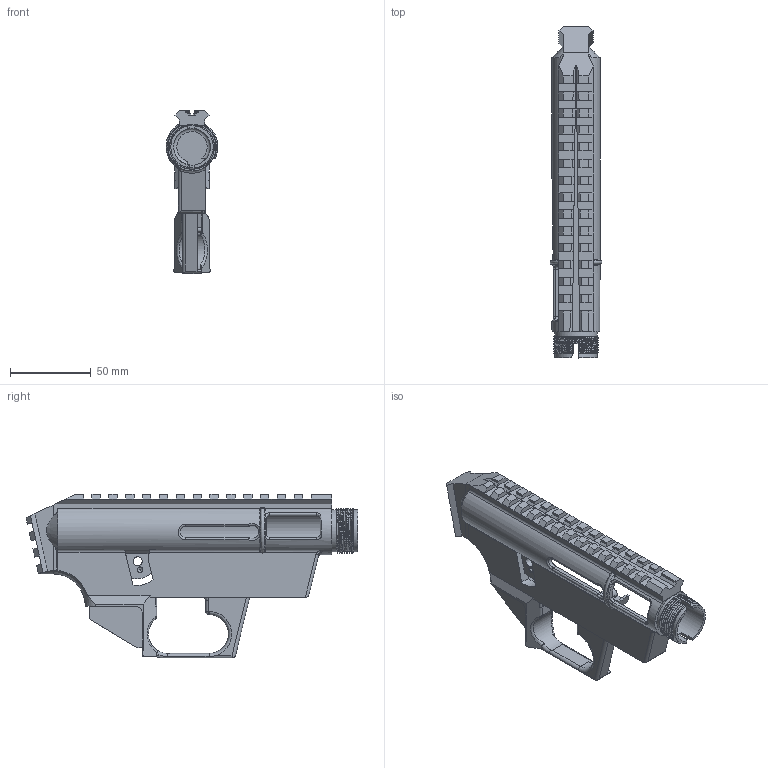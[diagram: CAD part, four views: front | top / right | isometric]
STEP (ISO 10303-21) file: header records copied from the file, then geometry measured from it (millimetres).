
FILE_DESCRIPTION(/* description */ (''),/* implementation_level */ '2;1');
FILE_NAME(/* name */ 'AR-7 Camper III v17.step',/* time_stamp */ '2021-02-13T00:44:38-05:00',/* author */ (''),/* organization */ (''),/* preprocessor_version */ 'ST-DEVELOPER v18.1',/* originating_system */ 'Autodesk Translation Framework v9.7.1.1290',/* authorisation */ '');
FILE_SCHEMA (('AUTOMOTIVE_DESIGN { 1 0 10303 214 3 1 1 }'));
Length unit declared in the file: millimetre
Products named in the file (1): AR-7 Camper III
Bounding box: 32.28 x 206.17 x 101.34 mm (x, y, z)
Volume: 134382.8 mm3; surface area: 55135.7 mm2
Topology: 3 solids, 3 shells, 590 faces, 1640 edges, 1053 vertices
Faces by surface type: plane 364, cylinder 128, bspline 63, torus 20, cone 11, sphere 4
Full cylindrical faces by diameter (mm): 3.45 x3, 3.65 x1, 4.3 x1, 5.5 x1, 5.65 x1, 7.75 x1, 22.9 x2, 26.132 x2, 26.3 x1, 27.85 x3
Entity records: 22740 total; most frequent: CARTESIAN_POINT 8004, ORIENTED_EDGE 3276, DIRECTION 2780, EDGE_CURVE 1638, LINE 1110, VECTOR 1110, VERTEX_POINT 1053, AXIS2_PLACEMENT_3D 835
